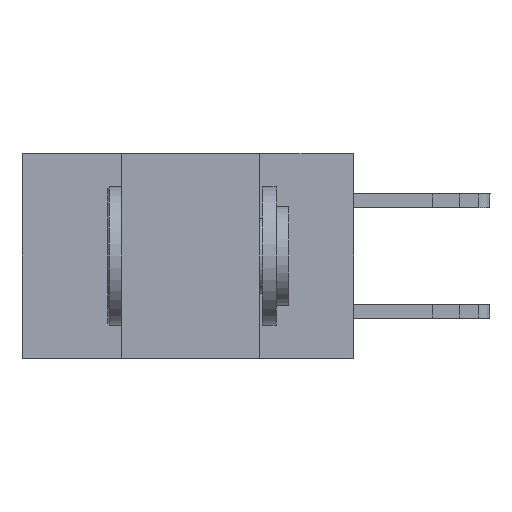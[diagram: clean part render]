
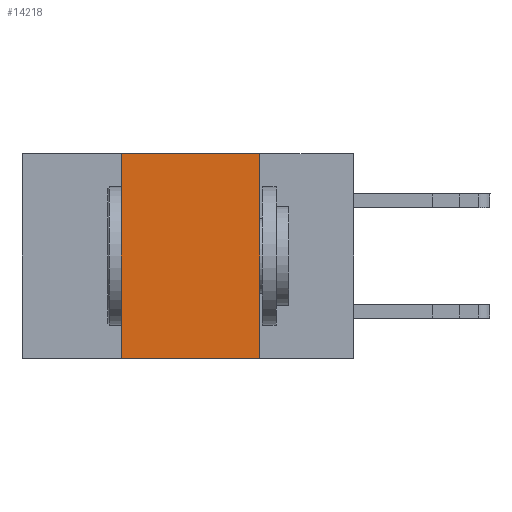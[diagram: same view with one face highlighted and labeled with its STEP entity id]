
A CAD part, left-side view. The second image highlights one B-rep face of the part: STEP entity #14218.
In plain terms, the highlighted planar face has unit normal (-1, 0, 0).
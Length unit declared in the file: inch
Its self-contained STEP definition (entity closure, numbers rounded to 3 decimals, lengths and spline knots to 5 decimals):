
#127 = EDGE_CURVE ( 'NONE', #278, #5970, #7167, .T. ) ;
#278 = VERTEX_POINT ( 'NONE', #17307 ) ;
#1629 = PLANE ( 'NONE',  #8648 ) ;
#2398 = VERTEX_POINT ( 'NONE', #6572 ) ;
#3628 = DIRECTION ( 'NONE',  ( 0., -1., 0. ) ) ;
#5159 = DIRECTION ( 'NONE',  ( 0., 0., -1. ) ) ;
#5527 = CARTESIAN_POINT ( 'NONE',  ( 0., 0.6, 0. ) ) ;
#5970 = VERTEX_POINT ( 'NONE', #8156 ) ;
#6312 = LINE ( 'NONE', #10994, #10803 ) ;
#6572 = CARTESIAN_POINT ( 'NONE',  ( 0., 0.17, -0.37 ) ) ;
#6870 = ORIENTED_EDGE ( 'NONE', *, *, #127, .F. ) ;
#6900 = ORIENTED_EDGE ( 'NONE', *, *, #20063, .F. ) ;
#7167 = LINE ( 'NONE', #5527, #22350 ) ;
#7804 = EDGE_CURVE ( 'NONE', #5970, #2398, #22592, .T. ) ;
#7988 = ORIENTED_EDGE ( 'NONE', *, *, #7804, .F. ) ;
#8156 = CARTESIAN_POINT ( 'NONE',  ( 0., 0.17, 0. ) ) ;
#8648 = AXIS2_PLACEMENT_3D ( 'NONE', #14177, #15829, #16062 ) ;
#9301 = CARTESIAN_POINT ( 'NONE',  ( 0., 0.42, -0.37 ) ) ;
#9589 = DIRECTION ( 'NONE',  ( 0., 0., 1. ) ) ;
#10803 = VECTOR ( 'NONE', #9589, 39.37008 ) ;
#10861 = VECTOR ( 'NONE', #21852, 39.37008 ) ;
#10994 = CARTESIAN_POINT ( 'NONE',  ( 0., 0.42, 0. ) ) ;
#11991 = EDGE_LOOP ( 'NONE', ( #7988, #6870, #6900, #14413 ) ) ;
#12980 = VECTOR ( 'NONE', #5159, 39.37008 ) ;
#13784 = VERTEX_POINT ( 'NONE', #9301 ) ;
#14177 = CARTESIAN_POINT ( 'NONE',  ( 0., 0.6, 0. ) ) ;
#14218 = ADVANCED_FACE ( 'NONE', ( #14916 ), #1629, .F. ) ;
#14413 = ORIENTED_EDGE ( 'NONE', *, *, #17803, .T. ) ;
#14779 = CARTESIAN_POINT ( 'NONE',  ( 0., 0.6, -0.37 ) ) ;
#14916 = FACE_OUTER_BOUND ( 'NONE', #11991, .T. ) ;
#15098 = LINE ( 'NONE', #14779, #10861 ) ;
#15829 = DIRECTION ( 'NONE',  ( 1., 0., 0. ) ) ;
#16062 = DIRECTION ( 'NONE',  ( 0., 0., -1. ) ) ;
#17307 = CARTESIAN_POINT ( 'NONE',  ( 0., 0.42, 0. ) ) ;
#17803 = EDGE_CURVE ( 'NONE', #13784, #2398, #15098, .T. ) ;
#20063 = EDGE_CURVE ( 'NONE', #13784, #278, #6312, .T. ) ;
#21033 = CARTESIAN_POINT ( 'NONE',  ( 0., 0.17, 0. ) ) ;
#21852 = DIRECTION ( 'NONE',  ( 0., -1., 0. ) ) ;
#22350 = VECTOR ( 'NONE', #3628, 39.37008 ) ;
#22592 = LINE ( 'NONE', #21033, #12980 ) ;
